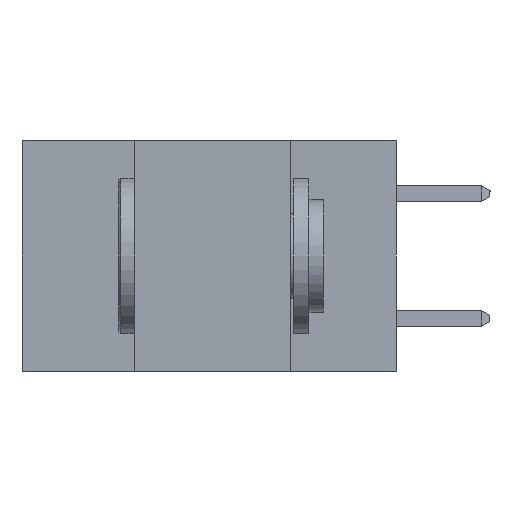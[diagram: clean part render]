
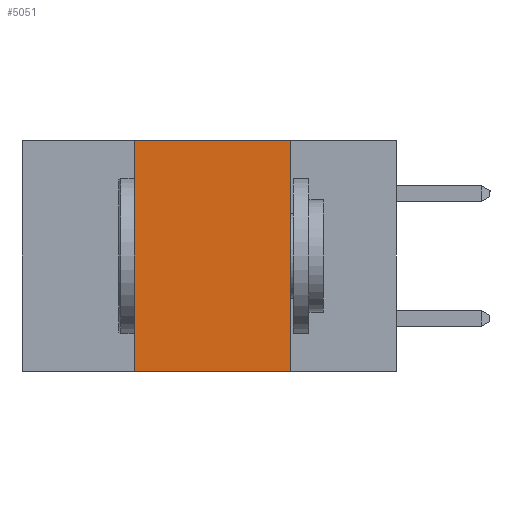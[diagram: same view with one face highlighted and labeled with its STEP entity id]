
A CAD part, left-side view. The second image highlights one B-rep face of the part: STEP entity #5051.
In plain terms, the highlighted planar face has unit normal (-1, 0, 0).
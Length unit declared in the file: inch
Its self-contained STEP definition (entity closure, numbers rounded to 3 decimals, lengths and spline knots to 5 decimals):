
#325 = FACE_OUTER_BOUND ( 'NONE', #12824, .T. ) ;
#1356 = CARTESIAN_POINT ( 'NONE',  ( 0., 0.42, 0. ) ) ;
#1844 = ORIENTED_EDGE ( 'NONE', *, *, #7813, .F. ) ;
#2270 = LINE ( 'NONE', #4689, #2767 ) ;
#2493 = VERTEX_POINT ( 'NONE', #1356 ) ;
#2572 = VECTOR ( 'NONE', #4136, 39.37008 ) ;
#2767 = VECTOR ( 'NONE', #17140, 39.37008 ) ;
#3716 = VERTEX_POINT ( 'NONE', #15606 ) ;
#4003 = VERTEX_POINT ( 'NONE', #12045 ) ;
#4136 = DIRECTION ( 'NONE',  ( 0., -1., 0. ) ) ;
#4689 = CARTESIAN_POINT ( 'NONE',  ( 0., 0.6, -0.37 ) ) ;
#4749 = CARTESIAN_POINT ( 'NONE',  ( 0., 0.17, 0. ) ) ;
#5051 = ADVANCED_FACE ( 'NONE', ( #325 ), #12450, .F. ) ;
#5150 = EDGE_CURVE ( 'NONE', #4003, #2493, #7372, .T. ) ;
#5615 = CARTESIAN_POINT ( 'NONE',  ( 0., 0.17, -0.37 ) ) ;
#5705 = DIRECTION ( 'NONE',  ( 0., 0., -1. ) ) ;
#6466 = EDGE_CURVE ( 'NONE', #4003, #3716, #2270, .T. ) ;
#6800 = EDGE_CURVE ( 'NONE', #2493, #7505, #10917, .T. ) ;
#7372 = LINE ( 'NONE', #11546, #12640 ) ;
#7505 = VERTEX_POINT ( 'NONE', #4749 ) ;
#7591 = ORIENTED_EDGE ( 'NONE', *, *, #6800, .F. ) ;
#7813 = EDGE_CURVE ( 'NONE', #7505, #3716, #9830, .T. ) ;
#8250 = DIRECTION ( 'NONE',  ( 0., 0., -1. ) ) ;
#8536 = ORIENTED_EDGE ( 'NONE', *, *, #6466, .T. ) ;
#9607 = DIRECTION ( 'NONE',  ( 1., 0., 0. ) ) ;
#9830 = LINE ( 'NONE', #5615, #11913 ) ;
#10917 = LINE ( 'NONE', #16316, #2572 ) ;
#11218 = ORIENTED_EDGE ( 'NONE', *, *, #5150, .F. ) ;
#11546 = CARTESIAN_POINT ( 'NONE',  ( 0., 0.42, -0.37 ) ) ;
#11913 = VECTOR ( 'NONE', #5705, 39.37008 ) ;
#12045 = CARTESIAN_POINT ( 'NONE',  ( 0., 0.42, -0.37 ) ) ;
#12357 = AXIS2_PLACEMENT_3D ( 'NONE', #12549, #9607, #8250 ) ;
#12450 = PLANE ( 'NONE',  #12357 ) ;
#12549 = CARTESIAN_POINT ( 'NONE',  ( 0., 0.6, 0. ) ) ;
#12640 = VECTOR ( 'NONE', #12886, 39.37008 ) ;
#12824 = EDGE_LOOP ( 'NONE', ( #1844, #7591, #11218, #8536 ) ) ;
#12886 = DIRECTION ( 'NONE',  ( 0., 0., 1. ) ) ;
#15606 = CARTESIAN_POINT ( 'NONE',  ( 0., 0.17, -0.37 ) ) ;
#16316 = CARTESIAN_POINT ( 'NONE',  ( 0., 0.6, 0. ) ) ;
#17140 = DIRECTION ( 'NONE',  ( 0., -1., 0. ) ) ;
